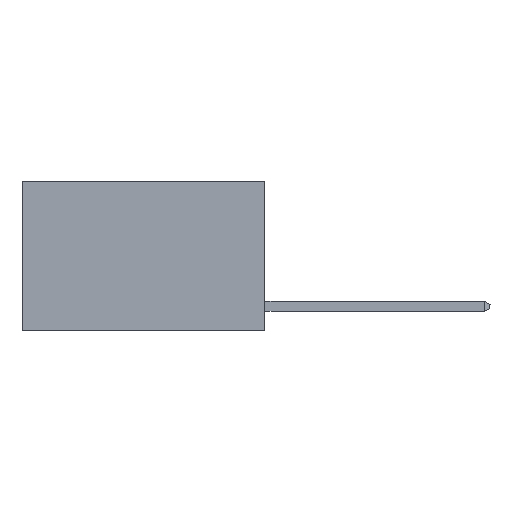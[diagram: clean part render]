
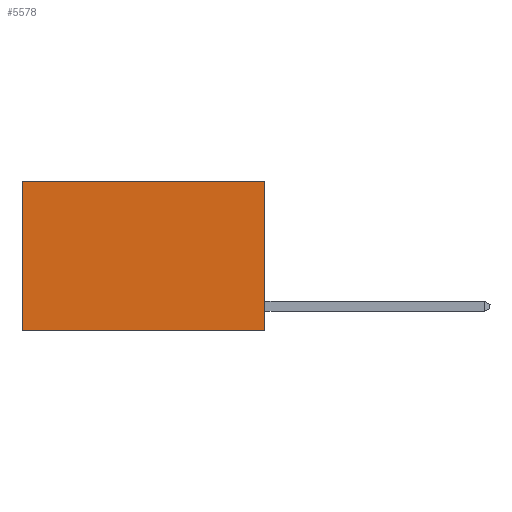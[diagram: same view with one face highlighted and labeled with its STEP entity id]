
A CAD part, left-side view. The second image highlights one B-rep face of the part: STEP entity #5578.
In plain terms, the highlighted planar face has unit normal (-1, 0, 0).
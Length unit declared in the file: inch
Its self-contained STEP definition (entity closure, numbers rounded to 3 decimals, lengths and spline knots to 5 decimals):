
#731 = DIRECTION ( 'NONE',  ( 0., 0., -1. ) ) ;
#1064 = VERTEX_POINT ( 'NONE', #5340 ) ;
#1321 = ORIENTED_EDGE ( 'NONE', *, *, #11887, .F. ) ;
#1889 = FACE_OUTER_BOUND ( 'NONE', #4218, .T. ) ;
#2088 = CARTESIAN_POINT ( 'NONE',  ( 0.2625, 0., 0. ) ) ;
#3154 = LINE ( 'NONE', #2088, #13273 ) ;
#3264 = VECTOR ( 'NONE', #4069, 39.37008 ) ;
#4066 = EDGE_CURVE ( 'NONE', #13425, #4849, #5815, .T. ) ;
#4069 = DIRECTION ( 'NONE',  ( 0., 1., 0. ) ) ;
#4218 = EDGE_LOOP ( 'NONE', ( #10106, #1321, #10774, #12285 ) ) ;
#4849 = VERTEX_POINT ( 'NONE', #11819 ) ;
#5340 = CARTESIAN_POINT ( 'NONE',  ( 0.2625, 0.6, -0.37 ) ) ;
#5578 = ADVANCED_FACE ( 'NONE', ( #1889 ), #9331, .F. ) ;
#5815 = LINE ( 'NONE', #6426, #8860 ) ;
#5883 = AXIS2_PLACEMENT_3D ( 'NONE', #8392, #8155, #13690 ) ;
#6015 = EDGE_CURVE ( 'NONE', #7601, #1064, #9317, .T. ) ;
#6166 = EDGE_CURVE ( 'NONE', #13425, #7601, #3154, .T. ) ;
#6426 = CARTESIAN_POINT ( 'NONE',  ( 0.2625, 0., 0. ) ) ;
#7601 = VERTEX_POINT ( 'NONE', #13066 ) ;
#8155 = DIRECTION ( 'NONE',  ( 1., 0., 0. ) ) ;
#8392 = CARTESIAN_POINT ( 'NONE',  ( 0.2625, 0., 0. ) ) ;
#8580 = LINE ( 'NONE', #13879, #3264 ) ;
#8860 = VECTOR ( 'NONE', #10874, 39.37008 ) ;
#9244 = CARTESIAN_POINT ( 'NONE',  ( 0.2625, 0.6, 0. ) ) ;
#9317 = LINE ( 'NONE', #9244, #11183 ) ;
#9331 = PLANE ( 'NONE',  #5883 ) ;
#9467 = CARTESIAN_POINT ( 'NONE',  ( 0.2625, 0., 0. ) ) ;
#10106 = ORIENTED_EDGE ( 'NONE', *, *, #6015, .T. ) ;
#10774 = ORIENTED_EDGE ( 'NONE', *, *, #4066, .F. ) ;
#10874 = DIRECTION ( 'NONE',  ( 0., 0., -1. ) ) ;
#11183 = VECTOR ( 'NONE', #731, 39.37008 ) ;
#11819 = CARTESIAN_POINT ( 'NONE',  ( 0.2625, 0., -0.37 ) ) ;
#11887 = EDGE_CURVE ( 'NONE', #4849, #1064, #8580, .T. ) ;
#12021 = DIRECTION ( 'NONE',  ( 0., 1., 0. ) ) ;
#12285 = ORIENTED_EDGE ( 'NONE', *, *, #6166, .T. ) ;
#13066 = CARTESIAN_POINT ( 'NONE',  ( 0.2625, 0.6, 0. ) ) ;
#13273 = VECTOR ( 'NONE', #12021, 39.37008 ) ;
#13425 = VERTEX_POINT ( 'NONE', #9467 ) ;
#13690 = DIRECTION ( 'NONE',  ( 0., 0., -1. ) ) ;
#13879 = CARTESIAN_POINT ( 'NONE',  ( 0.2625, 0., -0.37 ) ) ;
